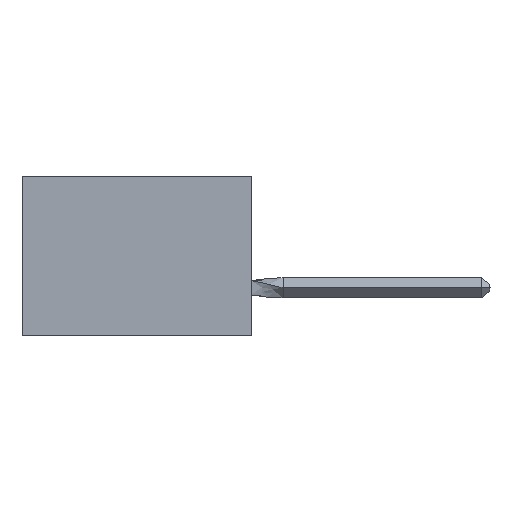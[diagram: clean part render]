
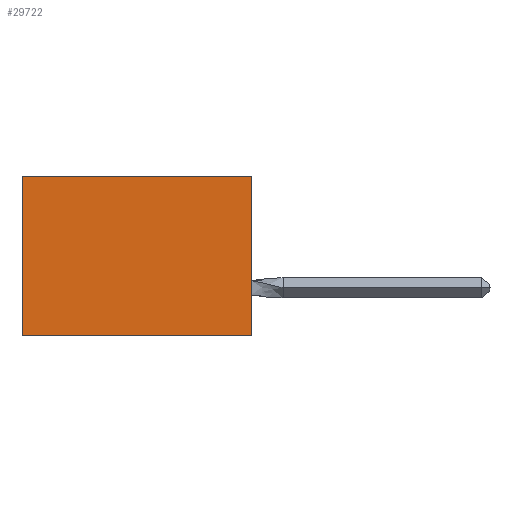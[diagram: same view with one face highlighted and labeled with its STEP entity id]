
A CAD part, left-side view. The second image highlights one B-rep face of the part: STEP entity #29722.
In plain terms, the highlighted planar face has unit normal (-1, 0, 0).
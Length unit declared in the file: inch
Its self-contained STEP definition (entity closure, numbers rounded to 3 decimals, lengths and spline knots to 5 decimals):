
#293 = CARTESIAN_POINT ( 'NONE',  ( 0.305, 0., -0.5 ) ) ;
#1628 = DIRECTION ( 'NONE',  ( 0., 0., -1. ) ) ;
#3099 = DIRECTION ( 'NONE',  ( 0., 1., 0. ) ) ;
#5660 = CARTESIAN_POINT ( 'NONE',  ( 0.305, 0., -0.5 ) ) ;
#7638 = ORIENTED_EDGE ( 'NONE', *, *, #29185, .F. ) ;
#8255 = EDGE_CURVE ( 'NONE', #9001, #17943, #31857, .T. ) ;
#9001 = VERTEX_POINT ( 'NONE', #10643 ) ;
#10129 = VECTOR ( 'NONE', #1628, 39.37008 ) ;
#10643 = CARTESIAN_POINT ( 'NONE',  ( 0.305, 0., 0. ) ) ;
#10826 = VERTEX_POINT ( 'NONE', #16146 ) ;
#11157 = ORIENTED_EDGE ( 'NONE', *, *, #18717, .T. ) ;
#11177 = DIRECTION ( 'NONE',  ( 0., 0., -1. ) ) ;
#11916 = VECTOR ( 'NONE', #18964, 39.37008 ) ;
#12107 = VERTEX_POINT ( 'NONE', #22669 ) ;
#12563 = EDGE_LOOP ( 'NONE', ( #11157, #7638, #17304, #20419 ) ) ;
#14194 = DIRECTION ( 'NONE',  ( 0., 0., -1. ) ) ;
#15812 = VECTOR ( 'NONE', #3099, 39.37008 ) ;
#16146 = CARTESIAN_POINT ( 'NONE',  ( 0.305, 0.72, -0.5 ) ) ;
#16744 = CARTESIAN_POINT ( 'NONE',  ( 0.305, 0., -0.5 ) ) ;
#16918 = LINE ( 'NONE', #16744, #27886 ) ;
#17304 = ORIENTED_EDGE ( 'NONE', *, *, #18550, .F. ) ;
#17943 = VERTEX_POINT ( 'NONE', #27148 ) ;
#18550 = EDGE_CURVE ( 'NONE', #9001, #12107, #16918, .T. ) ;
#18717 = EDGE_CURVE ( 'NONE', #17943, #10826, #26637, .T. ) ;
#18964 = DIRECTION ( 'NONE',  ( 0., 1., 0. ) ) ;
#20419 = ORIENTED_EDGE ( 'NONE', *, *, #8255, .T. ) ;
#22669 = CARTESIAN_POINT ( 'NONE',  ( 0.305, 0., -0.5 ) ) ;
#24302 = AXIS2_PLACEMENT_3D ( 'NONE', #293, #32530, #11177 ) ;
#25415 = LINE ( 'NONE', #5660, #11916 ) ;
#26637 = LINE ( 'NONE', #28858, #10129 ) ;
#27069 = FACE_OUTER_BOUND ( 'NONE', #12563, .T. ) ;
#27148 = CARTESIAN_POINT ( 'NONE',  ( 0.305, 0.72, 0. ) ) ;
#27886 = VECTOR ( 'NONE', #14194, 39.37008 ) ;
#28858 = CARTESIAN_POINT ( 'NONE',  ( 0.305, 0.72, -0.5 ) ) ;
#29185 = EDGE_CURVE ( 'NONE', #12107, #10826, #25415, .T. ) ;
#29722 = ADVANCED_FACE ( 'NONE', ( #27069 ), #30301, .F. ) ;
#30301 = PLANE ( 'NONE',  #24302 ) ;
#30611 = CARTESIAN_POINT ( 'NONE',  ( 0.305, 0., 0. ) ) ;
#31857 = LINE ( 'NONE', #30611, #15812 ) ;
#32530 = DIRECTION ( 'NONE',  ( 1., 0., 0. ) ) ;
